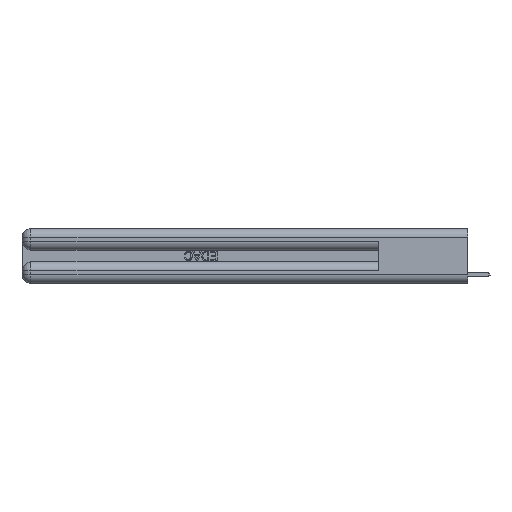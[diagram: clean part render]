
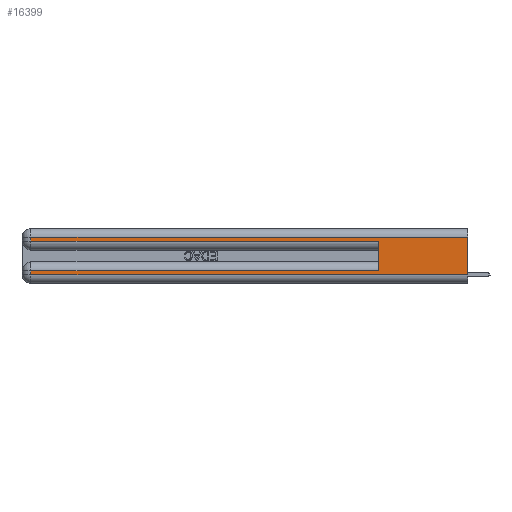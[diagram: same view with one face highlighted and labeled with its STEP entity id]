
A CAD part, left-side view. The second image highlights one B-rep face of the part: STEP entity #16399.
In plain terms, the highlighted planar face has unit normal (-1, 0, 0).
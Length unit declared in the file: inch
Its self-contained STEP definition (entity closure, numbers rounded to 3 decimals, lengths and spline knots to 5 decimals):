
#4 = AXIS2_PLACEMENT_3D ( 'NONE', #21025, #18148, #5945 ) ;
#503 = CARTESIAN_POINT ( 'NONE',  ( 0., 0., 0.06 ) ) ;
#1592 = LINE ( 'NONE', #11388, #16019 ) ;
#1823 = CARTESIAN_POINT ( 'NONE',  ( 0., 0.6, 0.285 ) ) ;
#2029 = EDGE_CURVE ( 'NONE', #8516, #30458, #21140, .T. ) ;
#2968 = VECTOR ( 'NONE', #4024, 39.37008 ) ;
#4024 = DIRECTION ( 'NONE',  ( 0., 1., 0. ) ) ;
#4650 = ORIENTED_EDGE ( 'NONE', *, *, #7796, .T. ) ;
#5019 = LINE ( 'NONE', #7425, #18312 ) ;
#5705 = VECTOR ( 'NONE', #16191, 39.37008 ) ;
#5758 = DIRECTION ( 'NONE',  ( 0., 0., -1. ) ) ;
#5945 = DIRECTION ( 'NONE',  ( 0., 0., -1. ) ) ;
#6703 = VECTOR ( 'NONE', #20783, 39.37008 ) ;
#6941 = ORIENTED_EDGE ( 'NONE', *, *, #11206, .T. ) ;
#7425 = CARTESIAN_POINT ( 'NONE',  ( 0., 0., 0.06 ) ) ;
#7796 = EDGE_CURVE ( 'NONE', #19825, #27988, #18226, .T. ) ;
#7953 = ORIENTED_EDGE ( 'NONE', *, *, #17766, .F. ) ;
#8469 = CARTESIAN_POINT ( 'NONE',  ( 0., 0., 0.285 ) ) ;
#8516 = VERTEX_POINT ( 'NONE', #14585 ) ;
#8675 = PLANE ( 'NONE',  #4 ) ;
#9073 = VERTEX_POINT ( 'NONE', #11807 ) ;
#9307 = LINE ( 'NONE', #19254, #2968 ) ;
#10141 = EDGE_CURVE ( 'NONE', #30179, #19825, #14873, .T. ) ;
#11206 = EDGE_CURVE ( 'NONE', #27988, #16153, #5019, .T. ) ;
#11388 = CARTESIAN_POINT ( 'NONE',  ( 0., 2.94, 0.37 ) ) ;
#11807 = CARTESIAN_POINT ( 'NONE',  ( 0., 2.94, 0.31 ) ) ;
#12190 = ORIENTED_EDGE ( 'NONE', *, *, #18671, .T. ) ;
#12667 = LINE ( 'NONE', #17799, #13405 ) ;
#13405 = VECTOR ( 'NONE', #5758, 39.37008 ) ;
#13646 = FACE_OUTER_BOUND ( 'NONE', #14105, .T. ) ;
#13771 = LINE ( 'NONE', #30465, #5705 ) ;
#14105 = EDGE_LOOP ( 'NONE', ( #7953, #28129, #12190, #18169, #15573, #21660, #4650, #6941 ) ) ;
#14585 = CARTESIAN_POINT ( 'NONE',  ( 0., 2.94, 0.285 ) ) ;
#14788 = CARTESIAN_POINT ( 'NONE',  ( 0., 0., 0.31 ) ) ;
#14806 = DIRECTION ( 'NONE',  ( 0., -1., 0. ) ) ;
#14873 = LINE ( 'NONE', #24641, #22887 ) ;
#15573 = ORIENTED_EDGE ( 'NONE', *, *, #17864, .F. ) ;
#15808 = CARTESIAN_POINT ( 'NONE',  ( 0., 2.94, 0.37 ) ) ;
#16019 = VECTOR ( 'NONE', #19225, 39.37008 ) ;
#16153 = VERTEX_POINT ( 'NONE', #503 ) ;
#16191 = DIRECTION ( 'NONE',  ( 0., 0., 1. ) ) ;
#16288 = CARTESIAN_POINT ( 'NONE',  ( 0., 2.94, 0.06 ) ) ;
#16399 = ADVANCED_FACE ( 'NONE', ( #13646 ), #8675, .F. ) ;
#17182 = VERTEX_POINT ( 'NONE', #14788 ) ;
#17766 = EDGE_CURVE ( 'NONE', #17182, #16153, #12667, .T. ) ;
#17799 = CARTESIAN_POINT ( 'NONE',  ( 0., 0., 0.37 ) ) ;
#17864 = EDGE_CURVE ( 'NONE', #30179, #30458, #13771, .T. ) ;
#18148 = DIRECTION ( 'NONE',  ( 1., 0., 0. ) ) ;
#18169 = ORIENTED_EDGE ( 'NONE', *, *, #2029, .T. ) ;
#18170 = CARTESIAN_POINT ( 'NONE',  ( 0., 2.94, 0.085 ) ) ;
#18226 = LINE ( 'NONE', #15808, #6703 ) ;
#18260 = DIRECTION ( 'NONE',  ( 0., -1., 0. ) ) ;
#18312 = VECTOR ( 'NONE', #14806, 39.37008 ) ;
#18671 = EDGE_CURVE ( 'NONE', #9073, #8516, #1592, .T. ) ;
#19225 = DIRECTION ( 'NONE',  ( 0., 0., -1. ) ) ;
#19254 = CARTESIAN_POINT ( 'NONE',  ( 0., 0., 0.31 ) ) ;
#19825 = VERTEX_POINT ( 'NONE', #18170 ) ;
#20783 = DIRECTION ( 'NONE',  ( 0., 0., -1. ) ) ;
#21025 = CARTESIAN_POINT ( 'NONE',  ( 0., 0., 0.37 ) ) ;
#21140 = LINE ( 'NONE', #8469, #30053 ) ;
#21660 = ORIENTED_EDGE ( 'NONE', *, *, #10141, .T. ) ;
#21929 = DIRECTION ( 'NONE',  ( 0., 1., 0. ) ) ;
#22887 = VECTOR ( 'NONE', #21929, 39.37008 ) ;
#23103 = EDGE_CURVE ( 'NONE', #17182, #9073, #9307, .T. ) ;
#24641 = CARTESIAN_POINT ( 'NONE',  ( 0., 0., 0.085 ) ) ;
#26602 = CARTESIAN_POINT ( 'NONE',  ( 0., 0.6, 0.085 ) ) ;
#27988 = VERTEX_POINT ( 'NONE', #16288 ) ;
#28129 = ORIENTED_EDGE ( 'NONE', *, *, #23103, .T. ) ;
#30053 = VECTOR ( 'NONE', #18260, 39.37008 ) ;
#30179 = VERTEX_POINT ( 'NONE', #26602 ) ;
#30458 = VERTEX_POINT ( 'NONE', #1823 ) ;
#30465 = CARTESIAN_POINT ( 'NONE',  ( 0., 0.6, 0.145 ) ) ;
